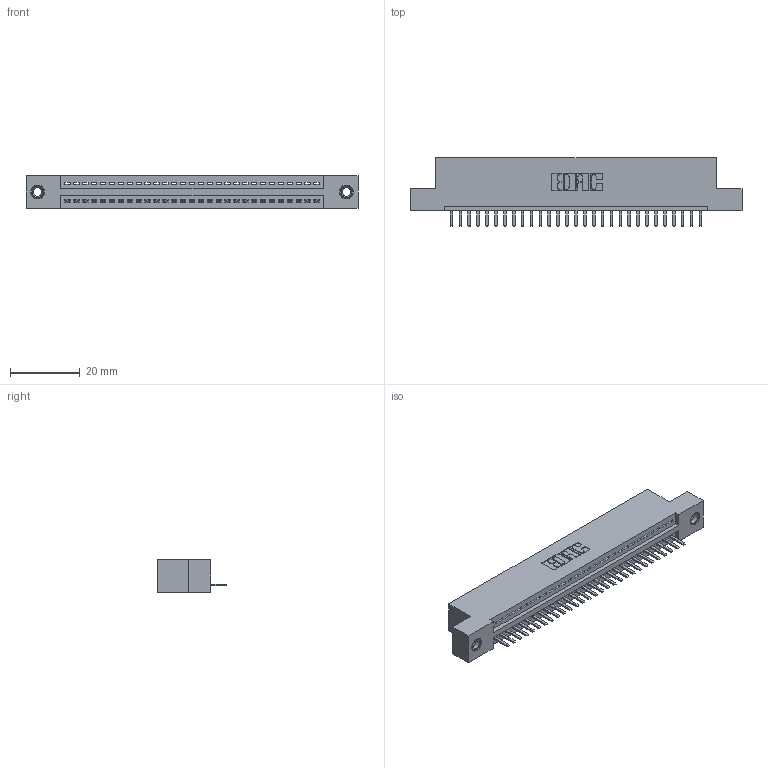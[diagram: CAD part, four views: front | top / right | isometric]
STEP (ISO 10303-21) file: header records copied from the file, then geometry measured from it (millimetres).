
FILE_DESCRIPTION (( 'STEP AP203' ), '1' );
FILE_NAME ('395-029-520-107.STEP', '2019-10-19T04:41:00', ( '' ), ( '' ), 'SwSTEP 2.0', 'SolidWorks 2016', '' );
FILE_SCHEMA (( 'CONFIG_CONTROL_DESIGN' ));
Length unit declared in the file: inch
Products named in the file (4): 345-292-001_345-293-120; 395-029-520-107; 345 Part_Flush Mounting Lugs - 0.156 Dia-TI; 345-250-001_345-250-005-103
Assembly tree (32 placements, depth 2):
  395-029-520-107
    345 Part_Flush Mounting Lugs - 0.156 Dia-TI
    345-292-001_345-293-120  x29
    345-250-001_345-250-005-103  x2
Bounding box: 94.87 x 19.68 x 9.4 mm (x, y, z)
Volume: 8807.3 mm3; surface area: 11287.1 mm2
Topology: 32 solids, 32 shells, 1984 faces, 5813 edges, 3790 vertices
Faces by surface type: plane 1330, cylinder 638, cone 12, torus 4
Entity records: 24876 total; most frequent: CARTESIAN_POINT 4302, ORIENTED_EDGE 4246, DIRECTION 3791, EDGE_CURVE 2123, VECTOR 1851, LINE 1851, VERTEX_POINT 1408, AXIS2_PLACEMENT_3D 970
